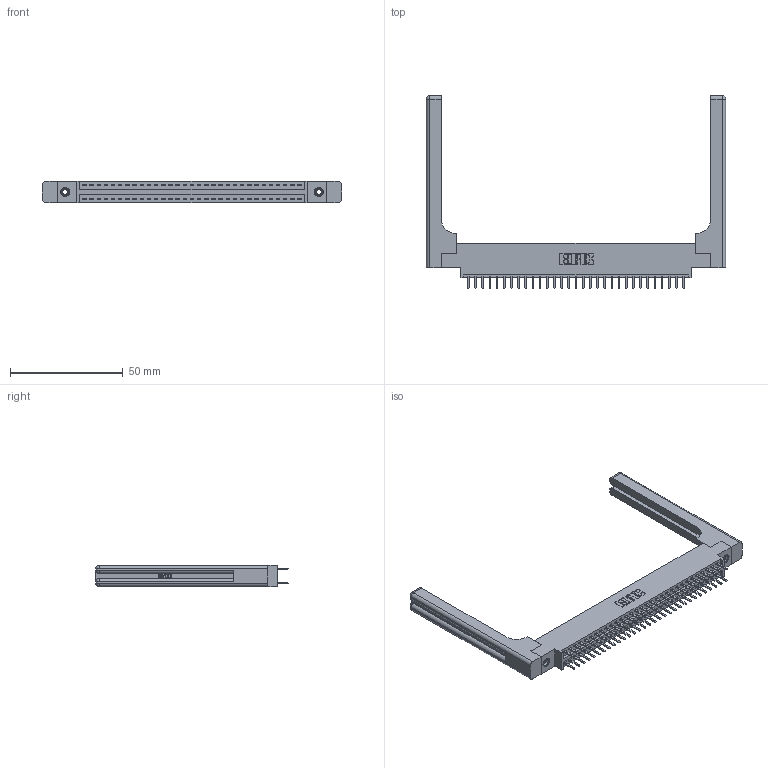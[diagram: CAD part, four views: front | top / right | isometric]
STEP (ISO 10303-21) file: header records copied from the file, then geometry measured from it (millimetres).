
FILE_DESCRIPTION (( 'STEP AP203' ), '1' );
FILE_NAME ('346-062-520-858.STEP', '2022-05-24T13:20:09', ( '' ), ( '' ), 'SwSTEP 2.0', 'SolidWorks 2020', '' );
FILE_SCHEMA (( 'CONFIG_CONTROL_DESIGN' ));
Length unit declared in the file: inch
Products named in the file (5): 345-250-001_345-250-001-102; 346-220-058_345-220-058; 346 Part_0.170 Offset - 0.156 Dia-TH; 346-062-520-858; 345-292-001_345-293-120
Assembly tree (67 placements, depth 2):
  346-062-520-858
    346 Part_0.170 Offset - 0.156 Dia-TH
    345-292-001_345-293-120  x62
    345-250-001_345-250-001-102  x2
    346-220-058_345-220-058  x2
Bounding box: 132.49 x 85.29 x 9.4 mm (x, y, z)
Volume: 20127.9 mm3; surface area: 22316 mm2
Topology: 67 solids, 67 shells, 3868 faces, 11149 edges, 7246 vertices
Faces by surface type: plane 2536, cylinder 1272, bspline 36, cone 12, sphere 8, torus 4
Entity records: 27556 total; most frequent: CARTESIAN_POINT 5583, ORIENTED_EDGE 4300, DIRECTION 3890, EDGE_CURVE 2150, LINE 1798, VECTOR 1798, VERTEX_POINT 1422, AXIS2_PLACEMENT_3D 1046
